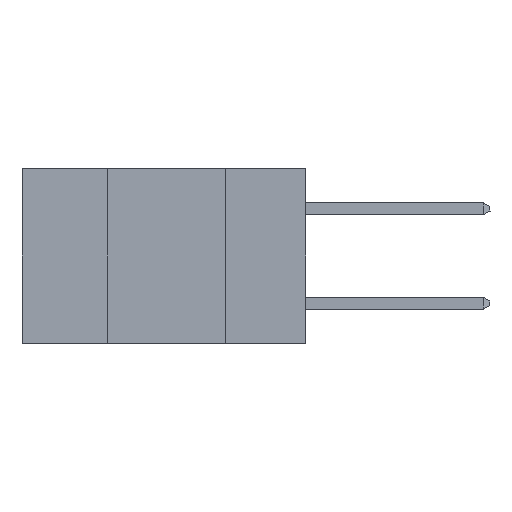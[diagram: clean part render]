
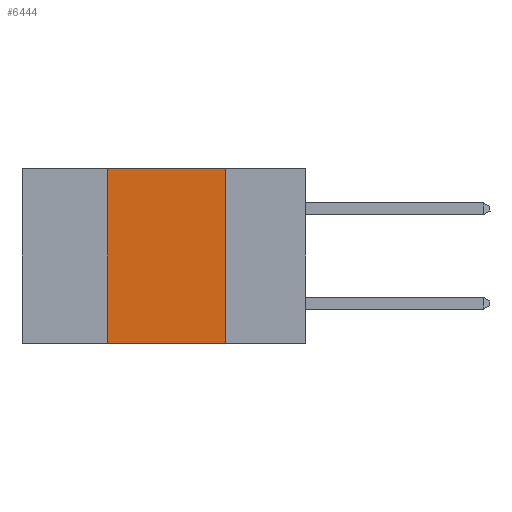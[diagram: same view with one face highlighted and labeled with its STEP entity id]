
A CAD part, left-side view. The second image highlights one B-rep face of the part: STEP entity #6444.
In plain terms, the highlighted planar face has unit normal (-1, 0, 0).
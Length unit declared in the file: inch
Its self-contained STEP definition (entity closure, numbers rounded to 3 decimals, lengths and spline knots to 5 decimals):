
#456 = VERTEX_POINT ( 'NONE', #5823 ) ;
#688 = LINE ( 'NONE', #7482, #9797 ) ;
#1483 = DIRECTION ( 'NONE',  ( 0., -1., 0. ) ) ;
#2218 = DIRECTION ( 'NONE',  ( 0., 0., -1. ) ) ;
#2555 = EDGE_CURVE ( 'NONE', #9816, #456, #6135, .T. ) ;
#2612 = CARTESIAN_POINT ( 'NONE',  ( 0., 0.42, 0. ) ) ;
#2765 = DIRECTION ( 'NONE',  ( 0., 0., -1. ) ) ;
#2896 = AXIS2_PLACEMENT_3D ( 'NONE', #7878, #5357, #2765 ) ;
#3902 = EDGE_CURVE ( 'NONE', #4606, #9816, #4583, .T. ) ;
#3998 = LINE ( 'NONE', #8420, #11132 ) ;
#4471 = EDGE_CURVE ( 'NONE', #4606, #7047, #3998, .T. ) ;
#4583 = LINE ( 'NONE', #4783, #10602 ) ;
#4606 = VERTEX_POINT ( 'NONE', #10387 ) ;
#4783 = CARTESIAN_POINT ( 'NONE',  ( 0., 0.42, 0. ) ) ;
#5145 = CARTESIAN_POINT ( 'NONE',  ( 0., 0.17, -0.37 ) ) ;
#5357 = DIRECTION ( 'NONE',  ( 1., 0., 0. ) ) ;
#5823 = CARTESIAN_POINT ( 'NONE',  ( 0., 0.17, 0. ) ) ;
#6135 = LINE ( 'NONE', #6259, #9837 ) ;
#6184 = PLANE ( 'NONE',  #2896 ) ;
#6238 = ORIENTED_EDGE ( 'NONE', *, *, #8238, .F. ) ;
#6259 = CARTESIAN_POINT ( 'NONE',  ( 0., 0.6, 0. ) ) ;
#6444 = ADVANCED_FACE ( 'NONE', ( #8519 ), #6184, .F. ) ;
#6728 = DIRECTION ( 'NONE',  ( 0., 0., 1. ) ) ;
#7047 = VERTEX_POINT ( 'NONE', #5145 ) ;
#7482 = CARTESIAN_POINT ( 'NONE',  ( 0., 0.17, 0. ) ) ;
#7878 = CARTESIAN_POINT ( 'NONE',  ( 0., 0.6, 0. ) ) ;
#8158 = ORIENTED_EDGE ( 'NONE', *, *, #3902, .F. ) ;
#8238 = EDGE_CURVE ( 'NONE', #456, #7047, #688, .T. ) ;
#8420 = CARTESIAN_POINT ( 'NONE',  ( 0., 0.6, -0.37 ) ) ;
#8519 = FACE_OUTER_BOUND ( 'NONE', #9071, .T. ) ;
#8892 = ORIENTED_EDGE ( 'NONE', *, *, #4471, .T. ) ;
#8907 = ORIENTED_EDGE ( 'NONE', *, *, #2555, .F. ) ;
#9005 = DIRECTION ( 'NONE',  ( 0., -1., 0. ) ) ;
#9071 = EDGE_LOOP ( 'NONE', ( #6238, #8907, #8158, #8892 ) ) ;
#9797 = VECTOR ( 'NONE', #2218, 39.37008 ) ;
#9816 = VERTEX_POINT ( 'NONE', #2612 ) ;
#9837 = VECTOR ( 'NONE', #9005, 39.37008 ) ;
#10387 = CARTESIAN_POINT ( 'NONE',  ( 0., 0.42, -0.37 ) ) ;
#10602 = VECTOR ( 'NONE', #6728, 39.37008 ) ;
#11132 = VECTOR ( 'NONE', #1483, 39.37008 ) ;
